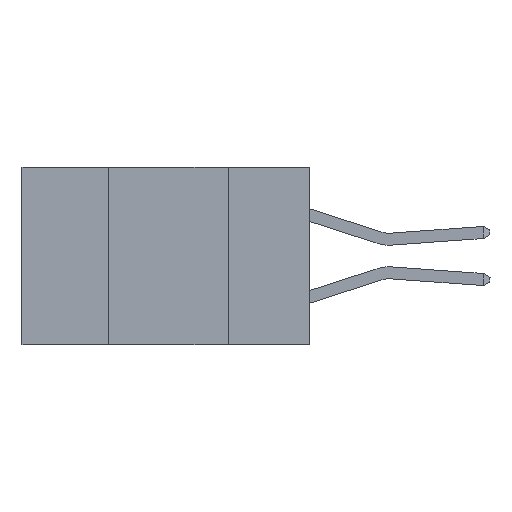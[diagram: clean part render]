
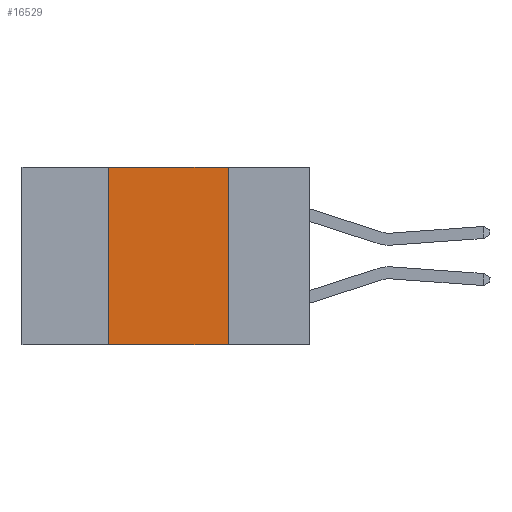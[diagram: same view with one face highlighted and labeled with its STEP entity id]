
A CAD part, left-side view. The second image highlights one B-rep face of the part: STEP entity #16529.
In plain terms, the highlighted planar face has unit normal (-1, 0, 0).
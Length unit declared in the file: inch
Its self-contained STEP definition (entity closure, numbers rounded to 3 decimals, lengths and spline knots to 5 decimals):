
#9 = CARTESIAN_POINT ( 'NONE',  ( 0., 0.17, 0. ) ) ;
#995 = ORIENTED_EDGE ( 'NONE', *, *, #18123, .F. ) ;
#1459 = ORIENTED_EDGE ( 'NONE', *, *, #3592, .F. ) ;
#1717 = ORIENTED_EDGE ( 'NONE', *, *, #20807, .T. ) ;
#1996 = EDGE_LOOP ( 'NONE', ( #995, #14599, #1459, #1717 ) ) ;
#2631 = DIRECTION ( 'NONE',  ( 0., 0., -1. ) ) ;
#2645 = AXIS2_PLACEMENT_3D ( 'NONE', #12530, #15960, #2631 ) ;
#3592 = EDGE_CURVE ( 'NONE', #13039, #19386, #7449, .T. ) ;
#3750 = CARTESIAN_POINT ( 'NONE',  ( 0., 0.42, -0.37 ) ) ;
#4364 = PLANE ( 'NONE',  #2645 ) ;
#7449 = LINE ( 'NONE', #19742, #11554 ) ;
#8590 = VERTEX_POINT ( 'NONE', #20735 ) ;
#9289 = DIRECTION ( 'NONE',  ( 0., 0., -1. ) ) ;
#10185 = LINE ( 'NONE', #11033, #17351 ) ;
#10299 = FACE_OUTER_BOUND ( 'NONE', #1996, .T. ) ;
#11033 = CARTESIAN_POINT ( 'NONE',  ( 0., 0.6, -0.37 ) ) ;
#11554 = VECTOR ( 'NONE', #13309, 39.37008 ) ;
#12245 = VECTOR ( 'NONE', #19827, 39.37008 ) ;
#12530 = CARTESIAN_POINT ( 'NONE',  ( 0., 0.6, 0. ) ) ;
#13039 = VERTEX_POINT ( 'NONE', #3750 ) ;
#13309 = DIRECTION ( 'NONE',  ( 0., 0., 1. ) ) ;
#13319 = CARTESIAN_POINT ( 'NONE',  ( 0., 0.6, 0. ) ) ;
#14510 = CARTESIAN_POINT ( 'NONE',  ( 0., 0.17, 0. ) ) ;
#14599 = ORIENTED_EDGE ( 'NONE', *, *, #20314, .F. ) ;
#15509 = VERTEX_POINT ( 'NONE', #9 ) ;
#15960 = DIRECTION ( 'NONE',  ( 1., 0., 0. ) ) ;
#16529 = ADVANCED_FACE ( 'NONE', ( #10299 ), #4364, .F. ) ;
#17131 = LINE ( 'NONE', #13319, #12245 ) ;
#17351 = VECTOR ( 'NONE', #21035, 39.37008 ) ;
#17388 = CARTESIAN_POINT ( 'NONE',  ( 0., 0.42, 0. ) ) ;
#17416 = VECTOR ( 'NONE', #9289, 39.37008 ) ;
#17912 = LINE ( 'NONE', #14510, #17416 ) ;
#18123 = EDGE_CURVE ( 'NONE', #15509, #8590, #17912, .T. ) ;
#19386 = VERTEX_POINT ( 'NONE', #17388 ) ;
#19742 = CARTESIAN_POINT ( 'NONE',  ( 0., 0.42, 0. ) ) ;
#19827 = DIRECTION ( 'NONE',  ( 0., -1., 0. ) ) ;
#20314 = EDGE_CURVE ( 'NONE', #19386, #15509, #17131, .T. ) ;
#20735 = CARTESIAN_POINT ( 'NONE',  ( 0., 0.17, -0.37 ) ) ;
#20807 = EDGE_CURVE ( 'NONE', #13039, #8590, #10185, .T. ) ;
#21035 = DIRECTION ( 'NONE',  ( 0., -1., 0. ) ) ;
